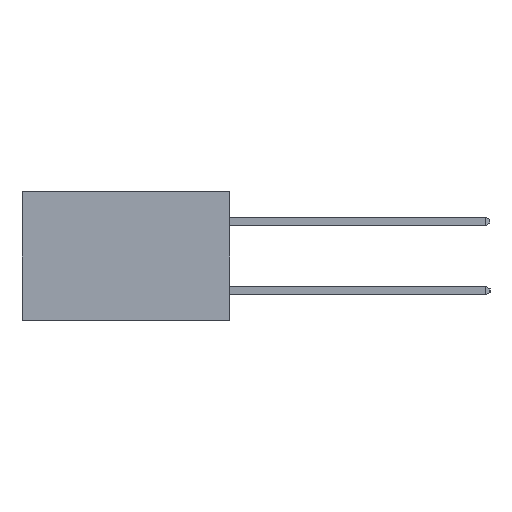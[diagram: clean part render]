
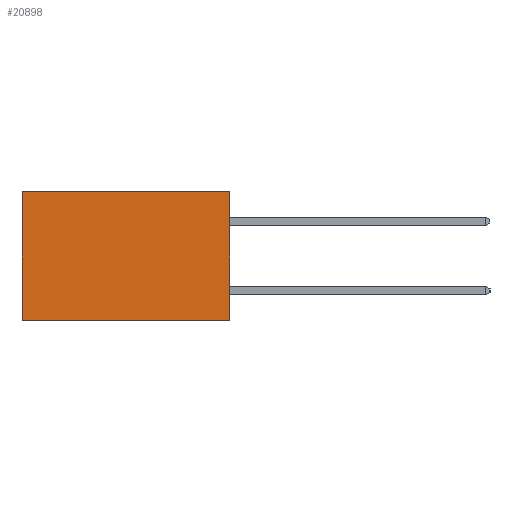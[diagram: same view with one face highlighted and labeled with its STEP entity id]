
A CAD part, left-side view. The second image highlights one B-rep face of the part: STEP entity #20898.
In plain terms, the highlighted planar face has unit normal (-1, 0, 0).
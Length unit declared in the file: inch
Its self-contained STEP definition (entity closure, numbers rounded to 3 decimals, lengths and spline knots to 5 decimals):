
#1166 = LINE ( 'NONE', #21997, #12037 ) ;
#1586 = CARTESIAN_POINT ( 'NONE',  ( 0.2615, 0.6, 0. ) ) ;
#1825 = DIRECTION ( 'NONE',  ( 0., 0., -1. ) ) ;
#2462 = CARTESIAN_POINT ( 'NONE',  ( 0.2615, 0., 0. ) ) ;
#2484 = VERTEX_POINT ( 'NONE', #5317 ) ;
#4165 = EDGE_CURVE ( 'NONE', #2484, #4799, #10574, .T. ) ;
#4256 = DIRECTION ( 'NONE',  ( 0., 0., -1. ) ) ;
#4799 = VERTEX_POINT ( 'NONE', #16489 ) ;
#5317 = CARTESIAN_POINT ( 'NONE',  ( 0.2615, 0., -0.37 ) ) ;
#6229 = VERTEX_POINT ( 'NONE', #2462 ) ;
#6518 = ORIENTED_EDGE ( 'NONE', *, *, #15569, .T. ) ;
#6573 = FACE_OUTER_BOUND ( 'NONE', #22118, .T. ) ;
#7966 = EDGE_CURVE ( 'NONE', #6229, #14006, #22952, .T. ) ;
#8601 = ORIENTED_EDGE ( 'NONE', *, *, #7966, .T. ) ;
#9734 = DIRECTION ( 'NONE',  ( 0., 1., 0. ) ) ;
#10400 = CARTESIAN_POINT ( 'NONE',  ( 0.2615, 0., -0.37 ) ) ;
#10574 = LINE ( 'NONE', #10400, #24510 ) ;
#10579 = DIRECTION ( 'NONE',  ( 0., 0., -1. ) ) ;
#11912 = CARTESIAN_POINT ( 'NONE',  ( 0.2615, 0., -0.37 ) ) ;
#12037 = VECTOR ( 'NONE', #10579, 39.37008 ) ;
#13061 = ORIENTED_EDGE ( 'NONE', *, *, #4165, .F. ) ;
#13373 = DIRECTION ( 'NONE',  ( 1., 0., 0. ) ) ;
#14006 = VERTEX_POINT ( 'NONE', #1586 ) ;
#14734 = LINE ( 'NONE', #11912, #24144 ) ;
#15287 = DIRECTION ( 'NONE',  ( 0., 1., 0. ) ) ;
#15569 = EDGE_CURVE ( 'NONE', #14006, #4799, #1166, .T. ) ;
#16064 = EDGE_CURVE ( 'NONE', #6229, #2484, #14734, .T. ) ;
#16216 = ORIENTED_EDGE ( 'NONE', *, *, #16064, .F. ) ;
#16489 = CARTESIAN_POINT ( 'NONE',  ( 0.2615, 0.6, -0.37 ) ) ;
#17945 = VECTOR ( 'NONE', #15287, 39.37008 ) ;
#20898 = ADVANCED_FACE ( 'NONE', ( #6573 ), #20931, .F. ) ;
#20931 = PLANE ( 'NONE',  #21910 ) ;
#21910 = AXIS2_PLACEMENT_3D ( 'NONE', #24662, #13373, #1825 ) ;
#21997 = CARTESIAN_POINT ( 'NONE',  ( 0.2615, 0.6, -0.37 ) ) ;
#22118 = EDGE_LOOP ( 'NONE', ( #6518, #13061, #16216, #8601 ) ) ;
#22952 = LINE ( 'NONE', #24642, #17945 ) ;
#24144 = VECTOR ( 'NONE', #4256, 39.37008 ) ;
#24510 = VECTOR ( 'NONE', #9734, 39.37008 ) ;
#24642 = CARTESIAN_POINT ( 'NONE',  ( 0.2615, 0., 0. ) ) ;
#24662 = CARTESIAN_POINT ( 'NONE',  ( 0.2615, 0., -0.37 ) ) ;
